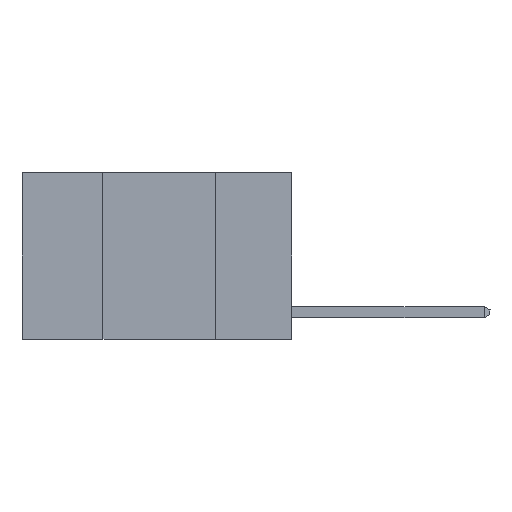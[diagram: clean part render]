
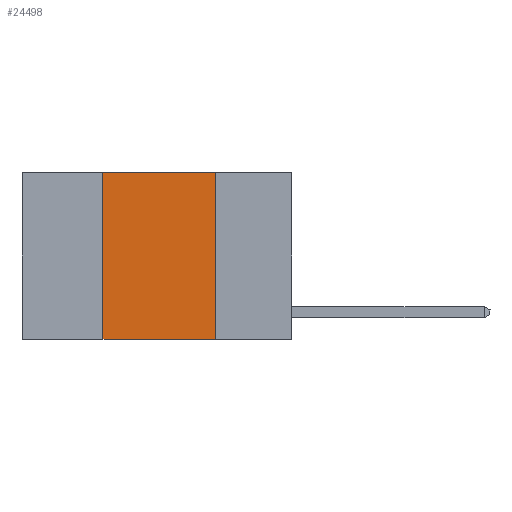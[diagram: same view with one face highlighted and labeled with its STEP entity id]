
A CAD part, left-side view. The second image highlights one B-rep face of the part: STEP entity #24498.
In plain terms, the highlighted planar face has unit normal (-1, 0, 0).
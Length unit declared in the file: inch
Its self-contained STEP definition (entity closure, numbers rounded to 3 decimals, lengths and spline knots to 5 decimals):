
#184 = DIRECTION ( 'NONE',  ( 0., -1., 0. ) ) ;
#473 = ORIENTED_EDGE ( 'NONE', *, *, #14787, .F. ) ;
#551 = DIRECTION ( 'NONE',  ( 0., 0., -1. ) ) ;
#3848 = EDGE_CURVE ( 'NONE', #27685, #6571, #19832, .T. ) ;
#3857 = CARTESIAN_POINT ( 'NONE',  ( 0., 0.17, -0.37 ) ) ;
#4521 = CARTESIAN_POINT ( 'NONE',  ( 0., 0.17, 0. ) ) ;
#5124 = CARTESIAN_POINT ( 'NONE',  ( 0., 0.6, 0. ) ) ;
#6571 = VERTEX_POINT ( 'NONE', #4521 ) ;
#7878 = VECTOR ( 'NONE', #184, 39.37008 ) ;
#8251 = EDGE_LOOP ( 'NONE', ( #22489, #16640, #473, #18976 ) ) ;
#9298 = EDGE_CURVE ( 'NONE', #22705, #18767, #15317, .T. ) ;
#9309 = VECTOR ( 'NONE', #13011, 39.37008 ) ;
#9638 = FACE_OUTER_BOUND ( 'NONE', #8251, .T. ) ;
#10333 = DIRECTION ( 'NONE',  ( 0., 0., 1. ) ) ;
#10421 = VECTOR ( 'NONE', #24695, 39.37008 ) ;
#10835 = EDGE_CURVE ( 'NONE', #6571, #18767, #11135, .T. ) ;
#11135 = LINE ( 'NONE', #18037, #10421 ) ;
#12008 = LINE ( 'NONE', #14788, #16609 ) ;
#13011 = DIRECTION ( 'NONE',  ( 0., -1., 0. ) ) ;
#14303 = DIRECTION ( 'NONE',  ( 1., 0., 0. ) ) ;
#14654 = AXIS2_PLACEMENT_3D ( 'NONE', #5124, #14303, #551 ) ;
#14787 = EDGE_CURVE ( 'NONE', #22705, #27685, #12008, .T. ) ;
#14788 = CARTESIAN_POINT ( 'NONE',  ( 0., 0.42, 0. ) ) ;
#15317 = LINE ( 'NONE', #17443, #9309 ) ;
#16468 = PLANE ( 'NONE',  #14654 ) ;
#16609 = VECTOR ( 'NONE', #10333, 39.37008 ) ;
#16640 = ORIENTED_EDGE ( 'NONE', *, *, #3848, .F. ) ;
#17443 = CARTESIAN_POINT ( 'NONE',  ( 0., 0.6, -0.37 ) ) ;
#18037 = CARTESIAN_POINT ( 'NONE',  ( 0., 0.17, 0. ) ) ;
#18767 = VERTEX_POINT ( 'NONE', #3857 ) ;
#18976 = ORIENTED_EDGE ( 'NONE', *, *, #9298, .T. ) ;
#19832 = LINE ( 'NONE', #27180, #7878 ) ;
#22489 = ORIENTED_EDGE ( 'NONE', *, *, #10835, .F. ) ;
#22705 = VERTEX_POINT ( 'NONE', #23619 ) ;
#23619 = CARTESIAN_POINT ( 'NONE',  ( 0., 0.42, -0.37 ) ) ;
#24498 = ADVANCED_FACE ( 'NONE', ( #9638 ), #16468, .F. ) ;
#24695 = DIRECTION ( 'NONE',  ( 0., 0., -1. ) ) ;
#27180 = CARTESIAN_POINT ( 'NONE',  ( 0., 0.6, 0. ) ) ;
#27258 = CARTESIAN_POINT ( 'NONE',  ( 0., 0.42, 0. ) ) ;
#27685 = VERTEX_POINT ( 'NONE', #27258 ) ;
